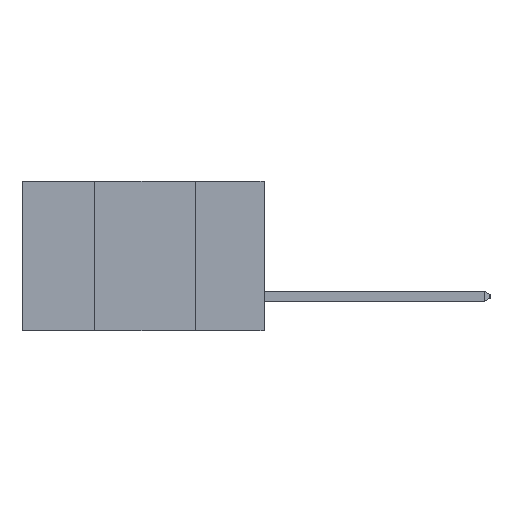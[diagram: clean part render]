
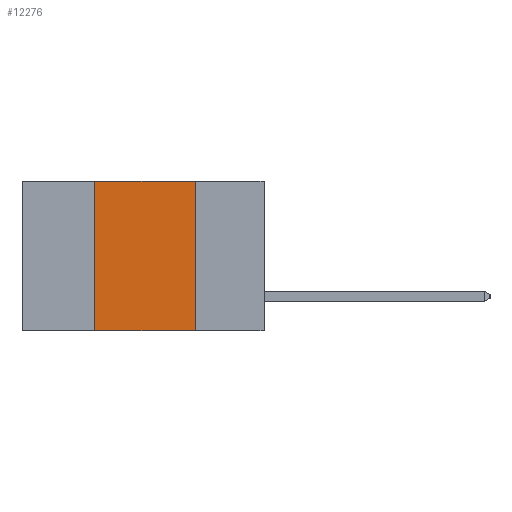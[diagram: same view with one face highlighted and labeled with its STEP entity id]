
A CAD part, left-side view. The second image highlights one B-rep face of the part: STEP entity #12276.
In plain terms, the highlighted planar face has unit normal (-1, 0, 0).
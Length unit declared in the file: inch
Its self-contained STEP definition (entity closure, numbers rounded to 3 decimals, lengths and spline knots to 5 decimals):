
#10 = DIRECTION ( 'NONE',  ( 0., -1., 0. ) ) ;
#48 = ORIENTED_EDGE ( 'NONE', *, *, #1151, .F. ) ;
#685 = VERTEX_POINT ( 'NONE', #8240 ) ;
#1151 = EDGE_CURVE ( 'NONE', #685, #16790, #8234, .T. ) ;
#1492 = CARTESIAN_POINT ( 'NONE',  ( 0., 0.17, -0.37 ) ) ;
#1494 = CARTESIAN_POINT ( 'NONE',  ( 0., 0.42, -0.37 ) ) ;
#3009 = CARTESIAN_POINT ( 'NONE',  ( 0., 0.6, -0.37 ) ) ;
#3560 = DIRECTION ( 'NONE',  ( 1., 0., 0. ) ) ;
#3637 = LINE ( 'NONE', #9962, #14406 ) ;
#3826 = VECTOR ( 'NONE', #13633, 39.37008 ) ;
#5123 = EDGE_CURVE ( 'NONE', #16790, #17515, #3637, .T. ) ;
#6044 = ORIENTED_EDGE ( 'NONE', *, *, #13363, .T. ) ;
#6239 = ORIENTED_EDGE ( 'NONE', *, *, #5123, .F. ) ;
#8145 = AXIS2_PLACEMENT_3D ( 'NONE', #18023, #3560, #13834 ) ;
#8234 = LINE ( 'NONE', #1494, #3826 ) ;
#8240 = CARTESIAN_POINT ( 'NONE',  ( 0., 0.42, -0.37 ) ) ;
#8661 = ORIENTED_EDGE ( 'NONE', *, *, #12037, .F. ) ;
#8757 = EDGE_LOOP ( 'NONE', ( #8661, #6239, #48, #6044 ) ) ;
#8889 = DIRECTION ( 'NONE',  ( 0., 0., -1. ) ) ;
#9198 = CARTESIAN_POINT ( 'NONE',  ( 0., 0.17, 0. ) ) ;
#9723 = DIRECTION ( 'NONE',  ( 0., -1., 0. ) ) ;
#9962 = CARTESIAN_POINT ( 'NONE',  ( 0., 0.6, 0. ) ) ;
#10063 = VECTOR ( 'NONE', #8889, 39.37008 ) ;
#10581 = CARTESIAN_POINT ( 'NONE',  ( 0., 0.42, 0. ) ) ;
#11197 = VECTOR ( 'NONE', #10, 39.37008 ) ;
#12037 = EDGE_CURVE ( 'NONE', #17515, #13062, #18093, .T. ) ;
#12276 = ADVANCED_FACE ( 'NONE', ( #17003 ), #16634, .F. ) ;
#13062 = VERTEX_POINT ( 'NONE', #15374 ) ;
#13363 = EDGE_CURVE ( 'NONE', #685, #13062, #17842, .T. ) ;
#13633 = DIRECTION ( 'NONE',  ( 0., 0., 1. ) ) ;
#13834 = DIRECTION ( 'NONE',  ( 0., 0., -1. ) ) ;
#14406 = VECTOR ( 'NONE', #9723, 39.37008 ) ;
#15374 = CARTESIAN_POINT ( 'NONE',  ( 0., 0.17, -0.37 ) ) ;
#16634 = PLANE ( 'NONE',  #8145 ) ;
#16790 = VERTEX_POINT ( 'NONE', #10581 ) ;
#17003 = FACE_OUTER_BOUND ( 'NONE', #8757, .T. ) ;
#17515 = VERTEX_POINT ( 'NONE', #9198 ) ;
#17842 = LINE ( 'NONE', #3009, #11197 ) ;
#18023 = CARTESIAN_POINT ( 'NONE',  ( 0., 0.6, 0. ) ) ;
#18093 = LINE ( 'NONE', #1492, #10063 ) ;
